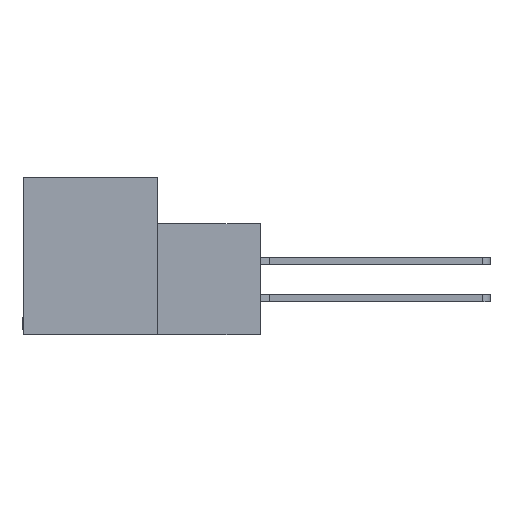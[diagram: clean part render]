
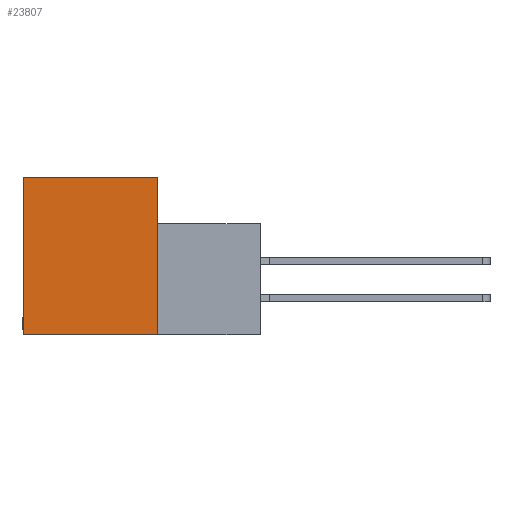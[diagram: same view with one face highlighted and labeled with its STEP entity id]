
A CAD part, left-side view. The second image highlights one B-rep face of the part: STEP entity #23807.
In plain terms, the highlighted planar face has unit normal (-1, 0, 0).
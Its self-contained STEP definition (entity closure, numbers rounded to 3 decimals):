
#270 = CARTESIAN_POINT ( 'NONE',  ( 0., 0., 0. ) ) ;
#390 = ORIENTED_EDGE ( 'NONE', *, *, #17618, .F. ) ;
#667 = EDGE_CURVE ( 'NONE', #12379, #21600, #8219, .T. ) ;
#1361 = CARTESIAN_POINT ( 'NONE',  ( 0., 0., -13.487 ) ) ;
#1798 = VERTEX_POINT ( 'NONE', #12564 ) ;
#2193 = AXIS2_PLACEMENT_3D ( 'NONE', #11820, #14126, #7957 ) ;
#4041 = DIRECTION ( 'NONE',  ( 0., 1., 0. ) ) ;
#6913 = CARTESIAN_POINT ( 'NONE',  ( 0., 0., 0. ) ) ;
#7279 = PLANE ( 'NONE',  #2193 ) ;
#7957 = DIRECTION ( 'NONE',  ( 0., 0., -1. ) ) ;
#8114 = EDGE_LOOP ( 'NONE', ( #390, #25636, #12631, #18663 ) ) ;
#8219 = LINE ( 'NONE', #6913, #21381 ) ;
#9522 = LINE ( 'NONE', #15215, #14859 ) ;
#10351 = DIRECTION ( 'NONE',  ( 0., -1., 0. ) ) ;
#11820 = CARTESIAN_POINT ( 'NONE',  ( 0., 0., 0. ) ) ;
#12379 = VERTEX_POINT ( 'NONE', #270 ) ;
#12564 = CARTESIAN_POINT ( 'NONE',  ( 0., 11.506, -13.487 ) ) ;
#12631 = ORIENTED_EDGE ( 'NONE', *, *, #13585, .F. ) ;
#13585 = EDGE_CURVE ( 'NONE', #27066, #12379, #9522, .T. ) ;
#14126 = DIRECTION ( 'NONE',  ( 1., 0., 0. ) ) ;
#14859 = VECTOR ( 'NONE', #10351, 1000. ) ;
#14870 = LINE ( 'NONE', #27024, #25480 ) ;
#15215 = CARTESIAN_POINT ( 'NONE',  ( 0., 11.506, 0. ) ) ;
#16143 = DIRECTION ( 'NONE',  ( 0., 0., -1. ) ) ;
#17510 = VECTOR ( 'NONE', #4041, 1000. ) ;
#17618 = EDGE_CURVE ( 'NONE', #21600, #1798, #18942, .T. ) ;
#18061 = CARTESIAN_POINT ( 'NONE',  ( 0., 11.506, 0. ) ) ;
#18663 = ORIENTED_EDGE ( 'NONE', *, *, #26371, .F. ) ;
#18942 = LINE ( 'NONE', #20194, #17510 ) ;
#20194 = CARTESIAN_POINT ( 'NONE',  ( 0., -8.814, -13.487 ) ) ;
#21381 = VECTOR ( 'NONE', #16143, 1000. ) ;
#21600 = VERTEX_POINT ( 'NONE', #1361 ) ;
#23807 = ADVANCED_FACE ( 'NONE', ( #24944 ), #7279, .F. ) ;
#24931 = DIRECTION ( 'NONE',  ( 0., 0., 1. ) ) ;
#24944 = FACE_OUTER_BOUND ( 'NONE', #8114, .T. ) ;
#25480 = VECTOR ( 'NONE', #24931, 1000. ) ;
#25636 = ORIENTED_EDGE ( 'NONE', *, *, #667, .F. ) ;
#26371 = EDGE_CURVE ( 'NONE', #1798, #27066, #14870, .T. ) ;
#27024 = CARTESIAN_POINT ( 'NONE',  ( 0., 11.506, -13.487 ) ) ;
#27066 = VERTEX_POINT ( 'NONE', #18061 ) ;
